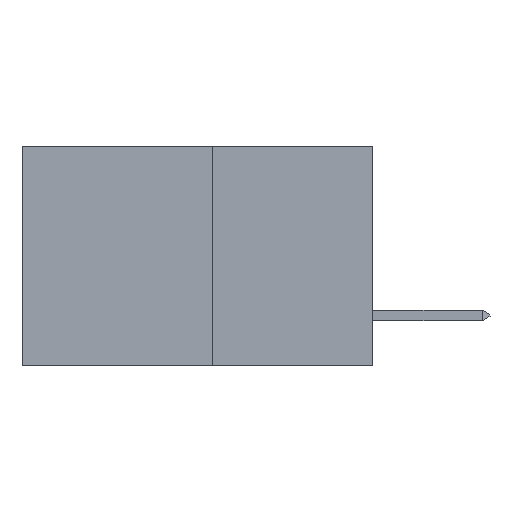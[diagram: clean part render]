
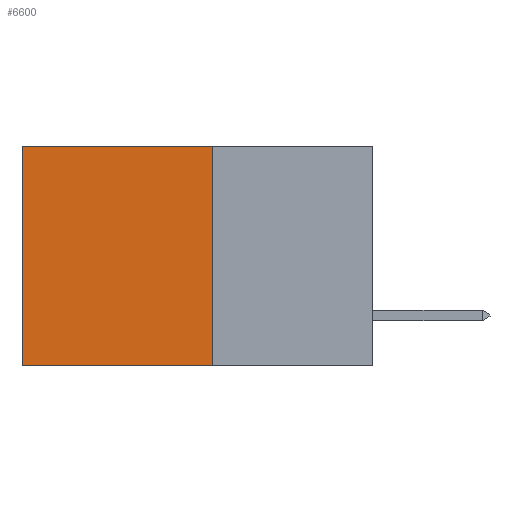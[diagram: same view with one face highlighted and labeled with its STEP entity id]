
A CAD part, left-side view. The second image highlights one B-rep face of the part: STEP entity #6600.
In plain terms, the highlighted planar face has unit normal (-1, 0, 0).
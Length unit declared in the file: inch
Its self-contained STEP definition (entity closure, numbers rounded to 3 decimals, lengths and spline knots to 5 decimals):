
#9 = FACE_OUTER_BOUND ( 'NONE', #633, .T. ) ;
#288 = ORIENTED_EDGE ( 'NONE', *, *, #7067, .T. ) ;
#411 = ORIENTED_EDGE ( 'NONE', *, *, #4239, .F. ) ;
#416 = CARTESIAN_POINT ( 'NONE',  ( 0.277, 0.27, -0.37 ) ) ;
#633 = EDGE_LOOP ( 'NONE', ( #288, #411, #10842, #10606 ) ) ;
#927 = DIRECTION ( 'NONE',  ( 0., 0., -1. ) ) ;
#1064 = CARTESIAN_POINT ( 'NONE',  ( 0.277, 0.59, 0. ) ) ;
#1084 = CARTESIAN_POINT ( 'NONE',  ( 0.277, 0.27, -0.37 ) ) ;
#1235 = VECTOR ( 'NONE', #8879, 39.37008 ) ;
#1430 = DIRECTION ( 'NONE',  ( 0., 0., -1. ) ) ;
#1519 = LINE ( 'NONE', #7770, #1235 ) ;
#1775 = VERTEX_POINT ( 'NONE', #8934 ) ;
#2296 = VECTOR ( 'NONE', #9085, 39.37008 ) ;
#2767 = VERTEX_POINT ( 'NONE', #1064 ) ;
#2816 = EDGE_CURVE ( 'NONE', #4553, #6188, #7278, .T. ) ;
#3103 = PLANE ( 'NONE',  #5449 ) ;
#3638 = CARTESIAN_POINT ( 'NONE',  ( 0.277, 0.27, 0. ) ) ;
#4152 = DIRECTION ( 'NONE',  ( 1., 0., 0. ) ) ;
#4239 = EDGE_CURVE ( 'NONE', #6188, #1775, #8798, .T. ) ;
#4260 = CARTESIAN_POINT ( 'NONE',  ( 0.277, 0.27, -0.37 ) ) ;
#4553 = VERTEX_POINT ( 'NONE', #3638 ) ;
#5057 = VECTOR ( 'NONE', #927, 39.37008 ) ;
#5449 = AXIS2_PLACEMENT_3D ( 'NONE', #4260, #4152, #1430 ) ;
#6188 = VERTEX_POINT ( 'NONE', #416 ) ;
#6600 = ADVANCED_FACE ( 'NONE', ( #9 ), #3103, .F. ) ;
#7067 = EDGE_CURVE ( 'NONE', #2767, #1775, #8890, .T. ) ;
#7224 = VECTOR ( 'NONE', #9903, 39.37008 ) ;
#7278 = LINE ( 'NONE', #1084, #5057 ) ;
#7770 = CARTESIAN_POINT ( 'NONE',  ( 0.277, 0.27, 0. ) ) ;
#8798 = LINE ( 'NONE', #8929, #2296 ) ;
#8879 = DIRECTION ( 'NONE',  ( 0., 1., 0. ) ) ;
#8890 = LINE ( 'NONE', #9952, #7224 ) ;
#8929 = CARTESIAN_POINT ( 'NONE',  ( 0.277, 0.27, -0.37 ) ) ;
#8934 = CARTESIAN_POINT ( 'NONE',  ( 0.277, 0.59, -0.37 ) ) ;
#9085 = DIRECTION ( 'NONE',  ( 0., 1., 0. ) ) ;
#9155 = EDGE_CURVE ( 'NONE', #4553, #2767, #1519, .T. ) ;
#9903 = DIRECTION ( 'NONE',  ( 0., 0., -1. ) ) ;
#9952 = CARTESIAN_POINT ( 'NONE',  ( 0.277, 0.59, -0.37 ) ) ;
#10606 = ORIENTED_EDGE ( 'NONE', *, *, #9155, .T. ) ;
#10842 = ORIENTED_EDGE ( 'NONE', *, *, #2816, .F. ) ;
